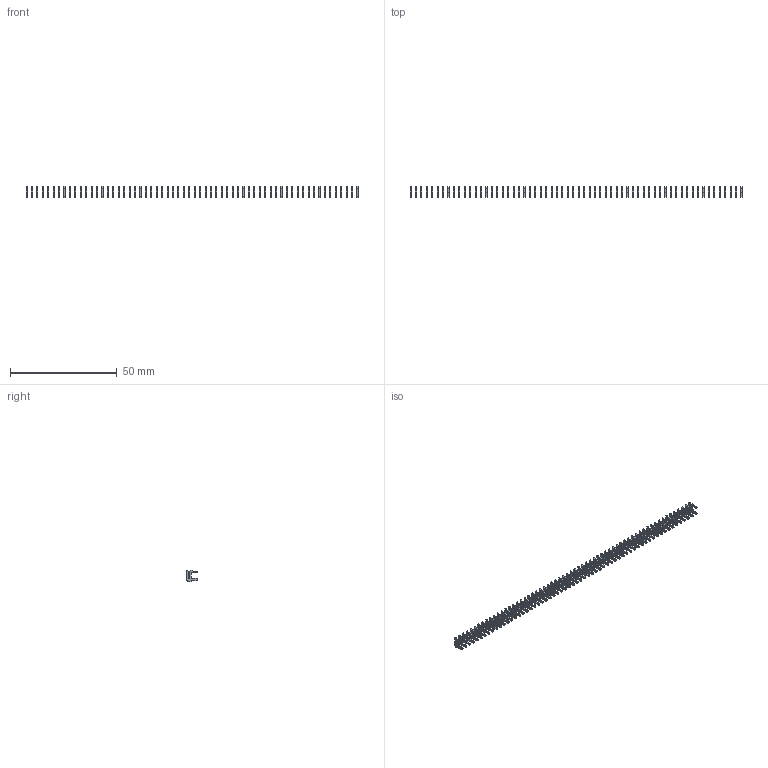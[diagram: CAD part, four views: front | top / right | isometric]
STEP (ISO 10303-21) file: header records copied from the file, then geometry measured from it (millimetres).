
FILE_DESCRIPTION (( 'STEP AP203' ), '1' );
FILE_NAME ('105-062-208-100.STEP', '2020-04-08T00:58:34', ( '' ), ( '' ), 'SwSTEP 2.0', 'SolidWorks 2016', '' );
FILE_SCHEMA (( 'CONFIG_CONTROL_DESIGN' ));
Length unit declared in the file: inch
Products named in the file (2): 105-062-208-100; 100-290-001_100-290-208
Assembly tree (62 placements, depth 2):
  105-062-208-100
    100-290-001_100-290-208  x62
Bounding box: 155.45 x 4.83 x 5.17 mm (x, y, z)
Volume: 426.6 mm3; surface area: 2634.8 mm2
Topology: 62 solids, 62 shells, 1550 faces, 4278 edges, 2852 vertices
Faces by surface type: plane 1364, cylinder 186
Entity records: 2941 total; most frequent: DIRECTION 255, CARTESIAN_POINT 205, ORIENTED_EDGE 138, LOCAL_TIME 134, COORDINATED_UNIVERSAL_TIME_OFFSET 134, CALENDAR_DATE 134, DATE_AND_TIME 134, AXIS2_PLACEMENT_3D 96
